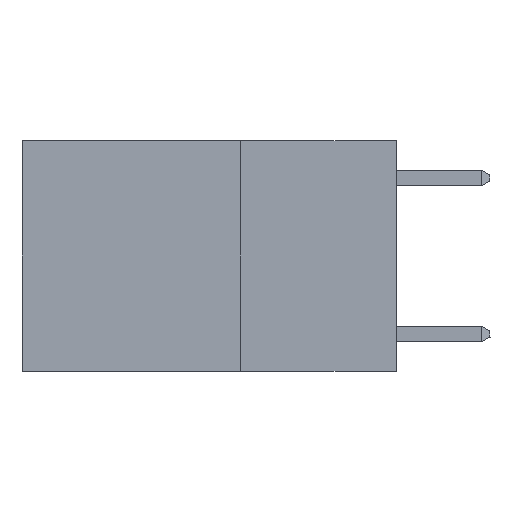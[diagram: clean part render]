
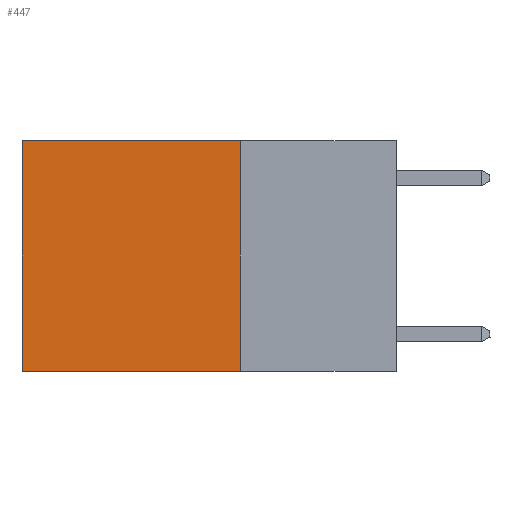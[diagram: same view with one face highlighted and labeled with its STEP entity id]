
A CAD part, left-side view. The second image highlights one B-rep face of the part: STEP entity #447.
In plain terms, the highlighted planar face has unit normal (-1, 0, 0).
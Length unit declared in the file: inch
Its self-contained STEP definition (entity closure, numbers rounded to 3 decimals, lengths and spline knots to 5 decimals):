
#447 = ADVANCED_FACE ( 'NONE', ( #1204 ), #9801, .F. ) ;
#622 = EDGE_CURVE ( 'NONE', #6206, #3711, #13291, .T. ) ;
#1204 = FACE_OUTER_BOUND ( 'NONE', #1668, .T. ) ;
#1425 = VERTEX_POINT ( 'NONE', #12706 ) ;
#1668 = EDGE_LOOP ( 'NONE', ( #8770, #13226, #6303, #7074 ) ) ;
#2214 = EDGE_CURVE ( 'NONE', #5334, #3711, #8030, .T. ) ;
#2575 = AXIS2_PLACEMENT_3D ( 'NONE', #5478, #9842, #3288 ) ;
#3040 = LINE ( 'NONE', #4962, #8552 ) ;
#3165 = VECTOR ( 'NONE', #4913, 39.37008 ) ;
#3288 = DIRECTION ( 'NONE',  ( 0., 0., -1. ) ) ;
#3711 = VERTEX_POINT ( 'NONE', #11131 ) ;
#4148 = DIRECTION ( 'NONE',  ( 0., 0., -1. ) ) ;
#4618 = EDGE_CURVE ( 'NONE', #1425, #6206, #6103, .T. ) ;
#4679 = CARTESIAN_POINT ( 'NONE',  ( 0.2625, 0.25, -0.37 ) ) ;
#4865 = CARTESIAN_POINT ( 'NONE',  ( 0.2625, 0.25, 0. ) ) ;
#4913 = DIRECTION ( 'NONE',  ( 0., 0., -1. ) ) ;
#4962 = CARTESIAN_POINT ( 'NONE',  ( 0.2625, 0.25, 0. ) ) ;
#5120 = VECTOR ( 'NONE', #4148, 39.37008 ) ;
#5334 = VERTEX_POINT ( 'NONE', #9027 ) ;
#5478 = CARTESIAN_POINT ( 'NONE',  ( 0.2625, 0.25, 0. ) ) ;
#6103 = LINE ( 'NONE', #4865, #3165 ) ;
#6206 = VERTEX_POINT ( 'NONE', #10662 ) ;
#6303 = ORIENTED_EDGE ( 'NONE', *, *, #4618, .F. ) ;
#7074 = ORIENTED_EDGE ( 'NONE', *, *, #11465, .T. ) ;
#7918 = VECTOR ( 'NONE', #12259, 39.37008 ) ;
#8030 = LINE ( 'NONE', #9652, #5120 ) ;
#8271 = DIRECTION ( 'NONE',  ( 0., 1., 0. ) ) ;
#8552 = VECTOR ( 'NONE', #8271, 39.37008 ) ;
#8770 = ORIENTED_EDGE ( 'NONE', *, *, #2214, .T. ) ;
#9027 = CARTESIAN_POINT ( 'NONE',  ( 0.2625, 0.6, 0. ) ) ;
#9652 = CARTESIAN_POINT ( 'NONE',  ( 0.2625, 0.6, 0. ) ) ;
#9801 = PLANE ( 'NONE',  #2575 ) ;
#9842 = DIRECTION ( 'NONE',  ( 1., 0., 0. ) ) ;
#10662 = CARTESIAN_POINT ( 'NONE',  ( 0.2625, 0.25, -0.37 ) ) ;
#11131 = CARTESIAN_POINT ( 'NONE',  ( 0.2625, 0.6, -0.37 ) ) ;
#11465 = EDGE_CURVE ( 'NONE', #1425, #5334, #3040, .T. ) ;
#12259 = DIRECTION ( 'NONE',  ( 0., 1., 0. ) ) ;
#12706 = CARTESIAN_POINT ( 'NONE',  ( 0.2625, 0.25, 0. ) ) ;
#13226 = ORIENTED_EDGE ( 'NONE', *, *, #622, .F. ) ;
#13291 = LINE ( 'NONE', #4679, #7918 ) ;
